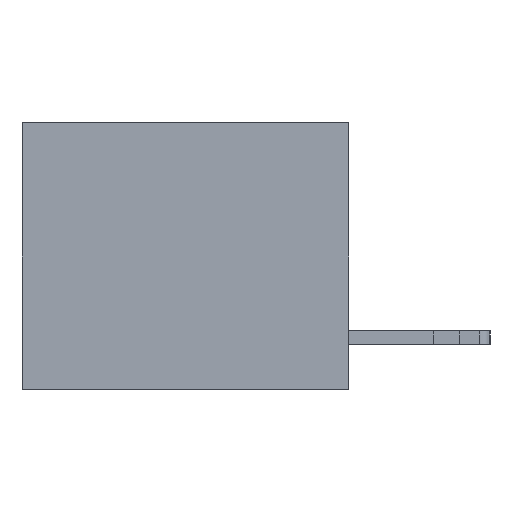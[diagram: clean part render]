
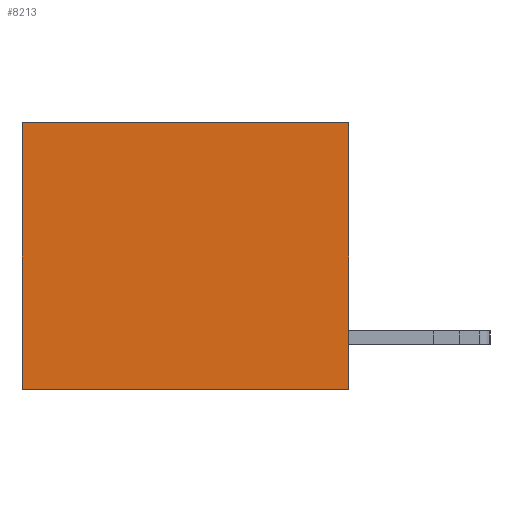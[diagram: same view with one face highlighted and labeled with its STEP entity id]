
A CAD part, left-side view. The second image highlights one B-rep face of the part: STEP entity #8213.
In plain terms, the highlighted planar face has unit normal (-1, 0, 0).
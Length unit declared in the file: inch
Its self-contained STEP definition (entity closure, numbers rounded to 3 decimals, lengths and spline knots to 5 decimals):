
#1012 = ORIENTED_EDGE ( 'NONE', *, *, #15560, .T. ) ;
#1446 = CARTESIAN_POINT ( 'NONE',  ( 0.3165, 0., 0. ) ) ;
#5662 = CARTESIAN_POINT ( 'NONE',  ( 0.3165, 0.6, -0.49 ) ) ;
#5764 = VECTOR ( 'NONE', #15806, 39.37008 ) ;
#6107 = CARTESIAN_POINT ( 'NONE',  ( 0.3165, 0., -0.49 ) ) ;
#6260 = AXIS2_PLACEMENT_3D ( 'NONE', #22804, #22888, #26790 ) ;
#7279 = CARTESIAN_POINT ( 'NONE',  ( 0.3165, 0., -0.49 ) ) ;
#7692 = ORIENTED_EDGE ( 'NONE', *, *, #19745, .F. ) ;
#8213 = ADVANCED_FACE ( 'NONE', ( #11391 ), #24661, .F. ) ;
#8981 = VERTEX_POINT ( 'NONE', #1446 ) ;
#9483 = CARTESIAN_POINT ( 'NONE',  ( 0.3165, 0.6, -0.49 ) ) ;
#9625 = LINE ( 'NONE', #7279, #19465 ) ;
#10170 = EDGE_CURVE ( 'NONE', #8981, #15753, #9625, .T. ) ;
#11391 = FACE_OUTER_BOUND ( 'NONE', #13636, .T. ) ;
#11506 = DIRECTION ( 'NONE',  ( 0., 0., -1. ) ) ;
#11514 = CARTESIAN_POINT ( 'NONE',  ( 0.3165, 0., 0. ) ) ;
#12353 = LINE ( 'NONE', #11514, #5764 ) ;
#13636 = EDGE_LOOP ( 'NONE', ( #1012, #7692, #13637, #19667 ) ) ;
#13637 = ORIENTED_EDGE ( 'NONE', *, *, #10170, .F. ) ;
#14146 = DIRECTION ( 'NONE',  ( 0., 0., -1. ) ) ;
#15560 = EDGE_CURVE ( 'NONE', #24502, #23054, #26998, .T. ) ;
#15753 = VERTEX_POINT ( 'NONE', #6107 ) ;
#15806 = DIRECTION ( 'NONE',  ( 0., 1., 0. ) ) ;
#17429 = CARTESIAN_POINT ( 'NONE',  ( 0.3165, 0., -0.49 ) ) ;
#17945 = LINE ( 'NONE', #17429, #22845 ) ;
#18757 = VECTOR ( 'NONE', #14146, 39.37008 ) ;
#19465 = VECTOR ( 'NONE', #11506, 39.37008 ) ;
#19667 = ORIENTED_EDGE ( 'NONE', *, *, #20391, .T. ) ;
#19745 = EDGE_CURVE ( 'NONE', #15753, #23054, #17945, .T. ) ;
#20391 = EDGE_CURVE ( 'NONE', #8981, #24502, #12353, .T. ) ;
#22561 = CARTESIAN_POINT ( 'NONE',  ( 0.3165, 0.6, 0. ) ) ;
#22804 = CARTESIAN_POINT ( 'NONE',  ( 0.3165, 0., -0.49 ) ) ;
#22845 = VECTOR ( 'NONE', #25679, 39.37008 ) ;
#22888 = DIRECTION ( 'NONE',  ( 1., 0., 0. ) ) ;
#23054 = VERTEX_POINT ( 'NONE', #9483 ) ;
#24502 = VERTEX_POINT ( 'NONE', #22561 ) ;
#24661 = PLANE ( 'NONE',  #6260 ) ;
#25679 = DIRECTION ( 'NONE',  ( 0., 1., 0. ) ) ;
#26790 = DIRECTION ( 'NONE',  ( 0., 0., -1. ) ) ;
#26998 = LINE ( 'NONE', #5662, #18757 ) ;
